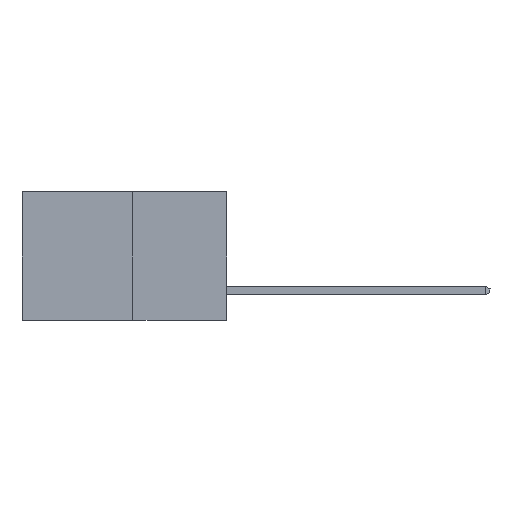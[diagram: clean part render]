
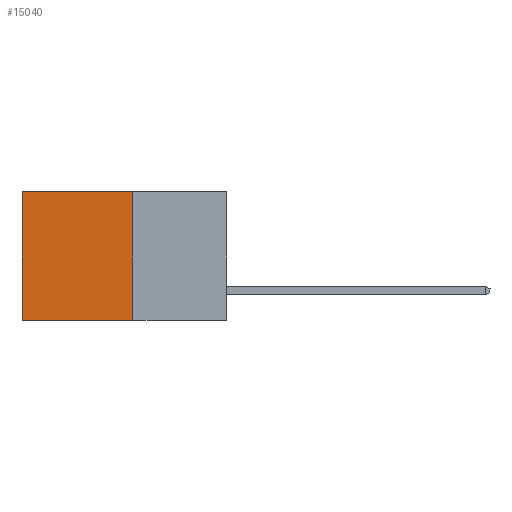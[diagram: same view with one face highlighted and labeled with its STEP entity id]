
A CAD part, left-side view. The second image highlights one B-rep face of the part: STEP entity #15040.
In plain terms, the highlighted planar face has unit normal (-1, 0, 0).
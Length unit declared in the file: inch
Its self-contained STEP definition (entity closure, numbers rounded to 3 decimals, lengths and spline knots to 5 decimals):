
#129 = VECTOR ( 'NONE', #11337, 39.37008 ) ;
#366 = CARTESIAN_POINT ( 'NONE',  ( 0.277, 0.27, -0.37 ) ) ;
#1260 = EDGE_CURVE ( 'NONE', #6367, #3426, #10081, .T. ) ;
#1882 = DIRECTION ( 'NONE',  ( 0., 0., -1. ) ) ;
#2187 = CARTESIAN_POINT ( 'NONE',  ( 0.277, 0.27, 0. ) ) ;
#2304 = ORIENTED_EDGE ( 'NONE', *, *, #3248, .T. ) ;
#2340 = ORIENTED_EDGE ( 'NONE', *, *, #1260, .F. ) ;
#2346 = EDGE_LOOP ( 'NONE', ( #2304, #2340, #2407, #2421 ) ) ;
#2407 = ORIENTED_EDGE ( 'NONE', *, *, #13017, .F. ) ;
#2421 = ORIENTED_EDGE ( 'NONE', *, *, #14749, .T. ) ;
#2602 = CARTESIAN_POINT ( 'NONE',  ( 0.277, 0.59, 0. ) ) ;
#2699 = CARTESIAN_POINT ( 'NONE',  ( 0.277, 0.27, -0.37 ) ) ;
#3248 = EDGE_CURVE ( 'NONE', #12692, #3426, #8006, .T. ) ;
#3266 = CARTESIAN_POINT ( 'NONE',  ( 0.277, 0.59, -0.37 ) ) ;
#3426 = VERTEX_POINT ( 'NONE', #3558 ) ;
#3480 = LINE ( 'NONE', #366, #9517 ) ;
#3558 = CARTESIAN_POINT ( 'NONE',  ( 0.277, 0.59, -0.37 ) ) ;
#4637 = CARTESIAN_POINT ( 'NONE',  ( 0.277, 0.27, 0. ) ) ;
#4747 = VECTOR ( 'NONE', #1882, 39.37008 ) ;
#4897 = AXIS2_PLACEMENT_3D ( 'NONE', #2699, #5162, #13444 ) ;
#5162 = DIRECTION ( 'NONE',  ( 1., 0., 0. ) ) ;
#5496 = FACE_OUTER_BOUND ( 'NONE', #2346, .T. ) ;
#6367 = VERTEX_POINT ( 'NONE', #9906 ) ;
#6713 = DIRECTION ( 'NONE',  ( 0., 0., -1. ) ) ;
#8006 = LINE ( 'NONE', #3266, #4747 ) ;
#9465 = DIRECTION ( 'NONE',  ( 0., 1., 0. ) ) ;
#9517 = VECTOR ( 'NONE', #6713, 39.37008 ) ;
#9685 = LINE ( 'NONE', #2187, #12407 ) ;
#9906 = CARTESIAN_POINT ( 'NONE',  ( 0.277, 0.27, -0.37 ) ) ;
#10081 = LINE ( 'NONE', #14459, #129 ) ;
#11337 = DIRECTION ( 'NONE',  ( 0., 1., 0. ) ) ;
#11538 = VERTEX_POINT ( 'NONE', #4637 ) ;
#12310 = PLANE ( 'NONE',  #4897 ) ;
#12407 = VECTOR ( 'NONE', #9465, 39.37008 ) ;
#12692 = VERTEX_POINT ( 'NONE', #2602 ) ;
#13017 = EDGE_CURVE ( 'NONE', #11538, #6367, #3480, .T. ) ;
#13444 = DIRECTION ( 'NONE',  ( 0., 0., -1. ) ) ;
#14459 = CARTESIAN_POINT ( 'NONE',  ( 0.277, 0.27, -0.37 ) ) ;
#14749 = EDGE_CURVE ( 'NONE', #11538, #12692, #9685, .T. ) ;
#15040 = ADVANCED_FACE ( 'NONE', ( #5496 ), #12310, .F. ) ;
